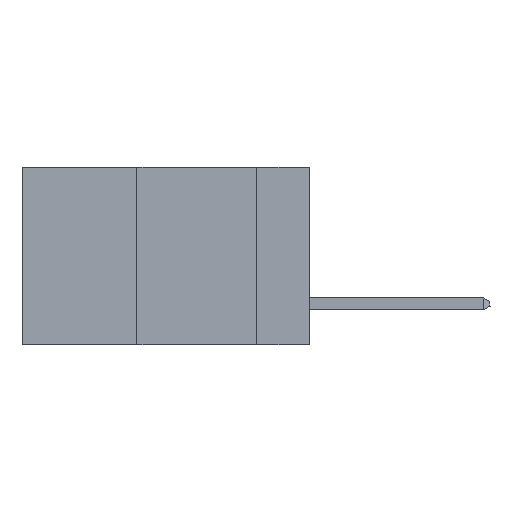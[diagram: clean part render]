
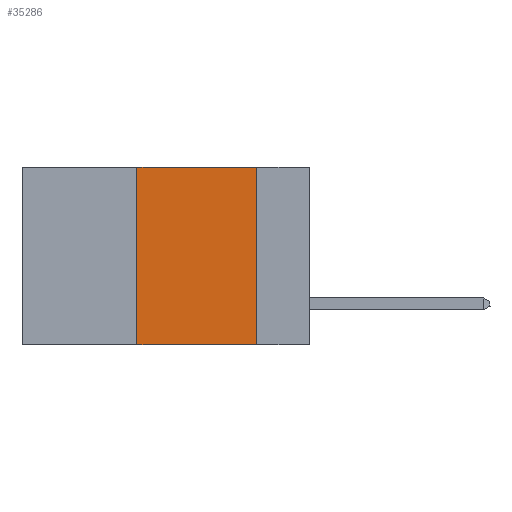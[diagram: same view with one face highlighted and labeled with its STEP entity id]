
A CAD part, left-side view. The second image highlights one B-rep face of the part: STEP entity #35286.
In plain terms, the highlighted planar face has unit normal (-1, 0, 0).
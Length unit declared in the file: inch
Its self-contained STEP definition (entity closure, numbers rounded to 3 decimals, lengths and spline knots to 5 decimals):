
#211 = DIRECTION ( 'NONE',  ( 0., 0., -1. ) ) ;
#913 = DIRECTION ( 'NONE',  ( 0., -1., 0. ) ) ;
#1267 = ORIENTED_EDGE ( 'NONE', *, *, #41761, .T. ) ;
#2827 = ORIENTED_EDGE ( 'NONE', *, *, #30816, .F. ) ;
#5105 = CARTESIAN_POINT ( 'NONE',  ( 0., 0.11, -0.37 ) ) ;
#5200 = AXIS2_PLACEMENT_3D ( 'NONE', #5731, #25338, #36522 ) ;
#5567 = PLANE ( 'NONE',  #5200 ) ;
#5731 = CARTESIAN_POINT ( 'NONE',  ( 0., 0.6, 0. ) ) ;
#7387 = CARTESIAN_POINT ( 'NONE',  ( 0., 0.11, 0. ) ) ;
#8123 = LINE ( 'NONE', #15818, #20158 ) ;
#8425 = EDGE_CURVE ( 'NONE', #37521, #48922, #48289, .T. ) ;
#12367 = EDGE_CURVE ( 'NONE', #48922, #25988, #47432, .T. ) ;
#15818 = CARTESIAN_POINT ( 'NONE',  ( 0., 0.11, 0. ) ) ;
#16698 = VECTOR ( 'NONE', #49964, 39.37008 ) ;
#20158 = VECTOR ( 'NONE', #211, 39.37008 ) ;
#22759 = CARTESIAN_POINT ( 'NONE',  ( 0., 0.36, 0. ) ) ;
#23759 = CARTESIAN_POINT ( 'NONE',  ( 0., 0.6, -0.37 ) ) ;
#24125 = CARTESIAN_POINT ( 'NONE',  ( 0., 0.36, 0. ) ) ;
#25338 = DIRECTION ( 'NONE',  ( 1., 0., 0. ) ) ;
#25670 = ORIENTED_EDGE ( 'NONE', *, *, #12367, .F. ) ;
#25988 = VERTEX_POINT ( 'NONE', #7387 ) ;
#27521 = CARTESIAN_POINT ( 'NONE',  ( 0., 0.6, 0. ) ) ;
#28008 = DIRECTION ( 'NONE',  ( 0., -1., 0. ) ) ;
#30816 = EDGE_CURVE ( 'NONE', #25988, #48362, #8123, .T. ) ;
#30874 = ORIENTED_EDGE ( 'NONE', *, *, #8425, .F. ) ;
#35172 = VECTOR ( 'NONE', #913, 39.37008 ) ;
#35286 = ADVANCED_FACE ( 'NONE', ( #37312 ), #5567, .F. ) ;
#36377 = LINE ( 'NONE', #23759, #35172 ) ;
#36522 = DIRECTION ( 'NONE',  ( 0., 0., -1. ) ) ;
#37312 = FACE_OUTER_BOUND ( 'NONE', #45077, .T. ) ;
#37521 = VERTEX_POINT ( 'NONE', #46400 ) ;
#41761 = EDGE_CURVE ( 'NONE', #37521, #48362, #36377, .T. ) ;
#45077 = EDGE_LOOP ( 'NONE', ( #2827, #25670, #30874, #1267 ) ) ;
#46400 = CARTESIAN_POINT ( 'NONE',  ( 0., 0.36, -0.37 ) ) ;
#47432 = LINE ( 'NONE', #27521, #48693 ) ;
#48289 = LINE ( 'NONE', #22759, #16698 ) ;
#48362 = VERTEX_POINT ( 'NONE', #5105 ) ;
#48693 = VECTOR ( 'NONE', #28008, 39.37008 ) ;
#48922 = VERTEX_POINT ( 'NONE', #24125 ) ;
#49964 = DIRECTION ( 'NONE',  ( 0., 0., 1. ) ) ;
